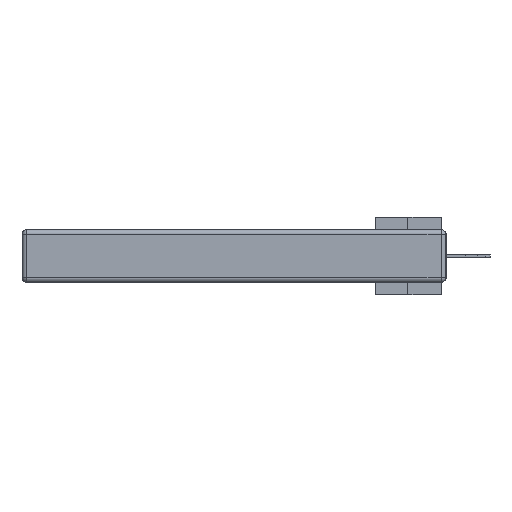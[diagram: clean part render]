
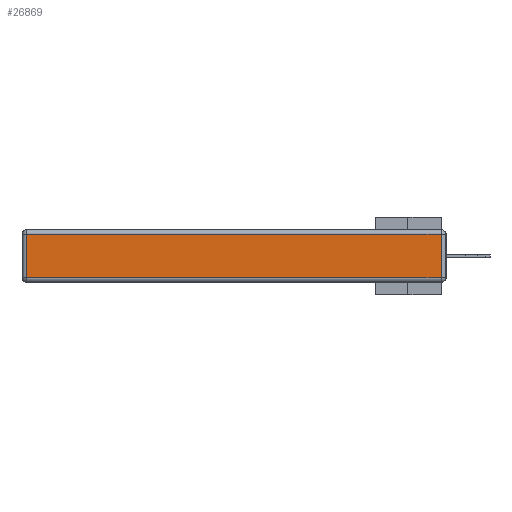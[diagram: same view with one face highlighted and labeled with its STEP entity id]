
A CAD part, left-side view. The second image highlights one B-rep face of the part: STEP entity #26869.
In plain terms, the highlighted planar face has unit normal (-1, 0, 0).
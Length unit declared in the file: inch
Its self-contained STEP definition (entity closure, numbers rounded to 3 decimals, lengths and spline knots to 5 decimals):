
#400 = CARTESIAN_POINT ( 'NONE',  ( 0., 0.03, -0.03 ) ) ;
#409 = DIRECTION ( 'NONE',  ( -1., 0., 0. ) ) ;
#1859 = DIRECTION ( 'NONE',  ( 0., -1., 0. ) ) ;
#2334 = CARTESIAN_POINT ( 'NONE',  ( 0., 2.72, -0.313 ) ) ;
#3693 = DIRECTION ( 'NONE',  ( 0., 0., -1. ) ) ;
#3771 = EDGE_CURVE ( 'NONE', #8281, #7217, #12896, .T. ) ;
#5848 = FACE_OUTER_BOUND ( 'NONE', #24184, .T. ) ;
#6230 = LINE ( 'NONE', #31840, #18894 ) ;
#7217 = VERTEX_POINT ( 'NONE', #2334 ) ;
#7926 = CARTESIAN_POINT ( 'NONE',  ( 0., 0.03, -0.343 ) ) ;
#8281 = VERTEX_POINT ( 'NONE', #20097 ) ;
#10472 = DIRECTION ( 'NONE',  ( 0., 0., 1. ) ) ;
#12896 = LINE ( 'NONE', #31152, #25380 ) ;
#15539 = CARTESIAN_POINT ( 'NONE',  ( 0., 0., -0.343 ) ) ;
#16174 = ORIENTED_EDGE ( 'NONE', *, *, #30611, .T. ) ;
#17766 = ORIENTED_EDGE ( 'NONE', *, *, #20677, .T. ) ;
#18117 = DIRECTION ( 'NONE',  ( 0., 0., 1. ) ) ;
#18894 = VECTOR ( 'NONE', #1859, 39.37008 ) ;
#19026 = LINE ( 'NONE', #7926, #31401 ) ;
#20006 = LINE ( 'NONE', #21359, #31614 ) ;
#20097 = CARTESIAN_POINT ( 'NONE',  ( 0., 2.72, -0.03 ) ) ;
#20677 = EDGE_CURVE ( 'NONE', #25068, #8281, #20006, .T. ) ;
#21244 = CARTESIAN_POINT ( 'NONE',  ( 0., 0.03, -0.313 ) ) ;
#21359 = CARTESIAN_POINT ( 'NONE',  ( 0., 2.75, -0.03 ) ) ;
#22775 = AXIS2_PLACEMENT_3D ( 'NONE', #15539, #409, #18117 ) ;
#23845 = DIRECTION ( 'NONE',  ( 0., 1., 0. ) ) ;
#24184 = EDGE_LOOP ( 'NONE', ( #27834, #16174, #17766, #25115 ) ) ;
#25068 = VERTEX_POINT ( 'NONE', #400 ) ;
#25115 = ORIENTED_EDGE ( 'NONE', *, *, #3771, .T. ) ;
#25380 = VECTOR ( 'NONE', #3693, 39.37008 ) ;
#26869 = ADVANCED_FACE ( 'NONE', ( #5848 ), #30340, .T. ) ;
#27027 = VERTEX_POINT ( 'NONE', #21244 ) ;
#27729 = EDGE_CURVE ( 'NONE', #7217, #27027, #6230, .T. ) ;
#27834 = ORIENTED_EDGE ( 'NONE', *, *, #27729, .T. ) ;
#30340 = PLANE ( 'NONE',  #22775 ) ;
#30611 = EDGE_CURVE ( 'NONE', #27027, #25068, #19026, .T. ) ;
#31152 = CARTESIAN_POINT ( 'NONE',  ( 0., 2.72, -0.343 ) ) ;
#31401 = VECTOR ( 'NONE', #10472, 39.37008 ) ;
#31614 = VECTOR ( 'NONE', #23845, 39.37008 ) ;
#31840 = CARTESIAN_POINT ( 'NONE',  ( 0., 0., -0.313 ) ) ;
